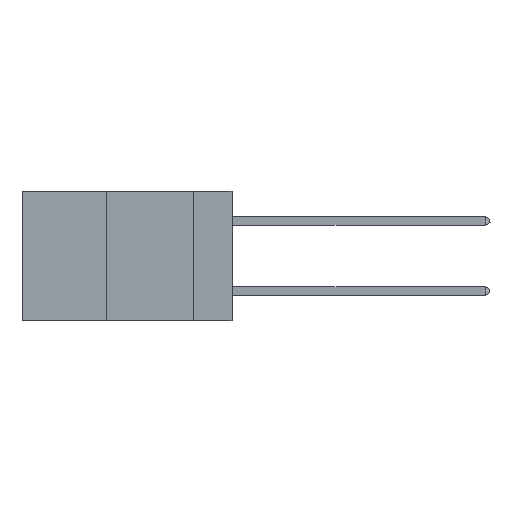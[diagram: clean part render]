
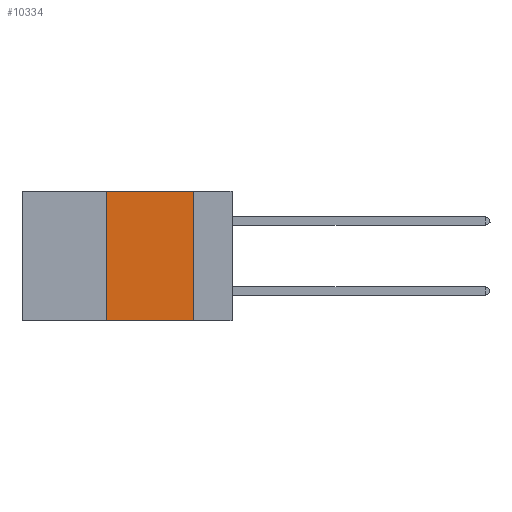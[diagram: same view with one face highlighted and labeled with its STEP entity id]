
A CAD part, left-side view. The second image highlights one B-rep face of the part: STEP entity #10334.
In plain terms, the highlighted planar face has unit normal (-1, 0, 0).
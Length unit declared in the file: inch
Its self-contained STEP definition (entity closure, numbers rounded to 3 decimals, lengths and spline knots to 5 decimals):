
#476 = LINE ( 'NONE', #6277, #16798 ) ;
#519 = ORIENTED_EDGE ( 'NONE', *, *, #4464, .F. ) ;
#697 = CARTESIAN_POINT ( 'NONE',  ( 0., 0.6, 0. ) ) ;
#812 = LINE ( 'NONE', #3711, #20274 ) ;
#1220 = VERTEX_POINT ( 'NONE', #12907 ) ;
#1808 = CARTESIAN_POINT ( 'NONE',  ( 0., 0.36, 0. ) ) ;
#2223 = FACE_OUTER_BOUND ( 'NONE', #2602, .T. ) ;
#2602 = EDGE_LOOP ( 'NONE', ( #16330, #8498, #519, #13157 ) ) ;
#3711 = CARTESIAN_POINT ( 'NONE',  ( 0., 0.6, -0.37 ) ) ;
#3967 = EDGE_CURVE ( 'NONE', #20120, #11094, #16390, .T. ) ;
#4464 = EDGE_CURVE ( 'NONE', #19015, #20120, #14905, .T. ) ;
#4597 = EDGE_CURVE ( 'NONE', #19015, #1220, #812, .T. ) ;
#5322 = DIRECTION ( 'NONE',  ( 0., -1., 0. ) ) ;
#6277 = CARTESIAN_POINT ( 'NONE',  ( 0., 0.11, 0. ) ) ;
#7059 = CARTESIAN_POINT ( 'NONE',  ( 0., 0.6, 0. ) ) ;
#7829 = DIRECTION ( 'NONE',  ( 0., 0., -1. ) ) ;
#8498 = ORIENTED_EDGE ( 'NONE', *, *, #3967, .F. ) ;
#8626 = DIRECTION ( 'NONE',  ( 0., -1., 0. ) ) ;
#9345 = EDGE_CURVE ( 'NONE', #11094, #1220, #476, .T. ) ;
#9693 = DIRECTION ( 'NONE',  ( 0., 0., 1. ) ) ;
#10194 = DIRECTION ( 'NONE',  ( 0., 0., -1. ) ) ;
#10334 = ADVANCED_FACE ( 'NONE', ( #2223 ), #18005, .F. ) ;
#11094 = VERTEX_POINT ( 'NONE', #15319 ) ;
#12907 = CARTESIAN_POINT ( 'NONE',  ( 0., 0.11, -0.37 ) ) ;
#13157 = ORIENTED_EDGE ( 'NONE', *, *, #4597, .T. ) ;
#14397 = VECTOR ( 'NONE', #9693, 39.37008 ) ;
#14818 = CARTESIAN_POINT ( 'NONE',  ( 0., 0.36, -0.37 ) ) ;
#14905 = LINE ( 'NONE', #1808, #14397 ) ;
#15319 = CARTESIAN_POINT ( 'NONE',  ( 0., 0.11, 0. ) ) ;
#16070 = CARTESIAN_POINT ( 'NONE',  ( 0., 0.36, 0. ) ) ;
#16330 = ORIENTED_EDGE ( 'NONE', *, *, #9345, .F. ) ;
#16390 = LINE ( 'NONE', #697, #20053 ) ;
#16798 = VECTOR ( 'NONE', #7829, 39.37008 ) ;
#17187 = AXIS2_PLACEMENT_3D ( 'NONE', #7059, #19576, #10194 ) ;
#18005 = PLANE ( 'NONE',  #17187 ) ;
#19015 = VERTEX_POINT ( 'NONE', #14818 ) ;
#19576 = DIRECTION ( 'NONE',  ( 1., 0., 0. ) ) ;
#20053 = VECTOR ( 'NONE', #8626, 39.37008 ) ;
#20120 = VERTEX_POINT ( 'NONE', #16070 ) ;
#20274 = VECTOR ( 'NONE', #5322, 39.37008 ) ;
